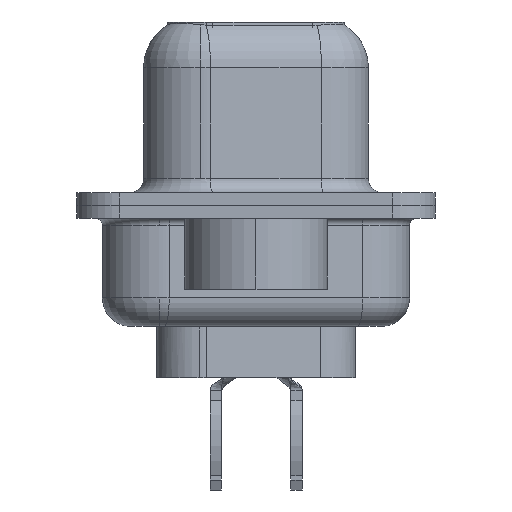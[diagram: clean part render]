
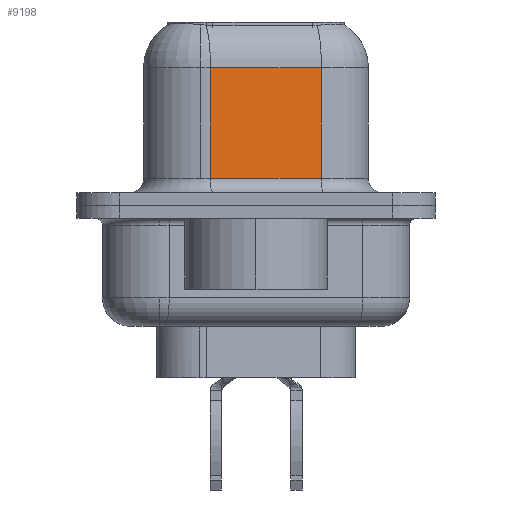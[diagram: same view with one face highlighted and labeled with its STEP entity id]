
A CAD part, left-side view. The second image highlights one B-rep face of the part: STEP entity #9198.
In plain terms, the highlighted planar face has unit normal (-0.985, -0.174, 0).
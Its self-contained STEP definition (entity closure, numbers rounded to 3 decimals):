
#8 = FACE_OUTER_BOUND ( 'NONE', #4425, .T. ) ;
#203 = LINE ( 'NONE', #3042, #1247 ) ;
#224 = CARTESIAN_POINT ( 'NONE',  ( 5.063, -2.297, 0.95 ) ) ;
#328 = EDGE_CURVE ( 'NONE', #11758, #1193, #7028, .T. ) ;
#1193 = VERTEX_POINT ( 'NONE', #16508 ) ;
#1247 = VECTOR ( 'NONE', #7678, 1000. ) ;
#1323 = DIRECTION ( 'NONE',  ( 0.985, 0.174, 0. ) ) ;
#3042 = CARTESIAN_POINT ( 'NONE',  ( 5.063, -2.297, 6.6 ) ) ;
#3180 = EDGE_CURVE ( 'NONE', #1193, #11402, #18087, .T. ) ;
#4425 = EDGE_LOOP ( 'NONE', ( #15982, #15800, #7755, #13159 ) ) ;
#5049 = VECTOR ( 'NONE', #10501, 1000. ) ;
#5650 = DIRECTION ( 'NONE',  ( -0.174, 0.985, 0. ) ) ;
#5988 = CARTESIAN_POINT ( 'NONE',  ( 5.063, -2.297, 0.95 ) ) ;
#7028 = LINE ( 'NONE', #19312, #16536 ) ;
#7492 = DIRECTION ( 'NONE',  ( -0.174, 0.985, 0. ) ) ;
#7678 = DIRECTION ( 'NONE',  ( 0., 0., -1. ) ) ;
#7755 = ORIENTED_EDGE ( 'NONE', *, *, #328, .T. ) ;
#8065 = AXIS2_PLACEMENT_3D ( 'NONE', #16841, #1323, #7492 ) ;
#9198 = ADVANCED_FACE ( 'NONE', ( #8 ), #14028, .F. ) ;
#9867 = CARTESIAN_POINT ( 'NONE',  ( 5.063, -2.297, 4.85 ) ) ;
#10501 = DIRECTION ( 'NONE',  ( 0.174, -0.985, 0. ) ) ;
#10541 = EDGE_CURVE ( 'NONE', #15302, #11758, #15018, .T. ) ;
#11402 = VERTEX_POINT ( 'NONE', #224 ) ;
#11681 = CARTESIAN_POINT ( 'NONE',  ( 5.063, -2.297, 4.85 ) ) ;
#11758 = VERTEX_POINT ( 'NONE', #15117 ) ;
#13159 = ORIENTED_EDGE ( 'NONE', *, *, #3180, .T. ) ;
#13935 = EDGE_CURVE ( 'NONE', #15302, #11402, #203, .T. ) ;
#14028 = PLANE ( 'NONE',  #8065 ) ;
#15018 = LINE ( 'NONE', #11681, #19731 ) ;
#15117 = CARTESIAN_POINT ( 'NONE',  ( 4.375, 1.603, 4.85 ) ) ;
#15302 = VERTEX_POINT ( 'NONE', #9867 ) ;
#15800 = ORIENTED_EDGE ( 'NONE', *, *, #10541, .T. ) ;
#15982 = ORIENTED_EDGE ( 'NONE', *, *, #13935, .F. ) ;
#16382 = DIRECTION ( 'NONE',  ( 0., 0., -1. ) ) ;
#16508 = CARTESIAN_POINT ( 'NONE',  ( 4.375, 1.603, 0.95 ) ) ;
#16536 = VECTOR ( 'NONE', #16382, 1000. ) ;
#16841 = CARTESIAN_POINT ( 'NONE',  ( 5.063, -2.297, 6.6 ) ) ;
#18087 = LINE ( 'NONE', #5988, #5049 ) ;
#19312 = CARTESIAN_POINT ( 'NONE',  ( 4.375, 1.603, 6.6 ) ) ;
#19731 = VECTOR ( 'NONE', #5650, 1000. ) ;
